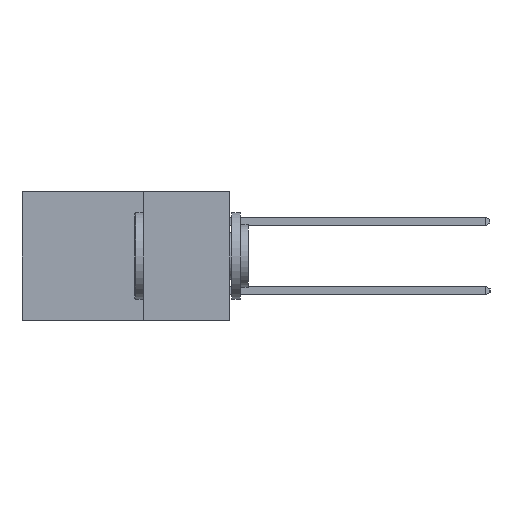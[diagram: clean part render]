
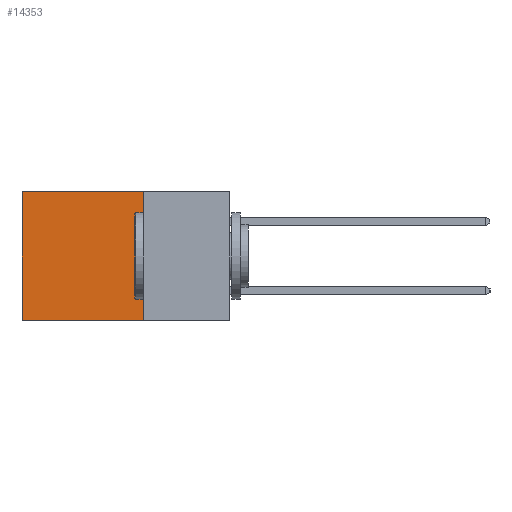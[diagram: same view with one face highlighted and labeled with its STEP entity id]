
A CAD part, left-side view. The second image highlights one B-rep face of the part: STEP entity #14353.
In plain terms, the highlighted planar face has unit normal (-1, 0, 0).
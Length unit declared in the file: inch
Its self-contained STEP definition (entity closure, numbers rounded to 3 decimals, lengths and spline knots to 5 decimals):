
#50 = ORIENTED_EDGE ( 'NONE', *, *, #10143, .T. ) ;
#382 = VECTOR ( 'NONE', #13634, 39.37008 ) ;
#398 = VECTOR ( 'NONE', #5019, 39.37008 ) ;
#512 = CARTESIAN_POINT ( 'NONE',  ( 0.2615, 0.6, -0.37 ) ) ;
#1094 = VECTOR ( 'NONE', #5701, 39.37008 ) ;
#2653 = ORIENTED_EDGE ( 'NONE', *, *, #5101, .F. ) ;
#3463 = CARTESIAN_POINT ( 'NONE',  ( 0.2615, 0.25, -0.37 ) ) ;
#4507 = FACE_OUTER_BOUND ( 'NONE', #9122, .T. ) ;
#4672 = VERTEX_POINT ( 'NONE', #5315 ) ;
#4679 = LINE ( 'NONE', #512, #382 ) ;
#5019 = DIRECTION ( 'NONE',  ( 0., 1., 0. ) ) ;
#5101 = EDGE_CURVE ( 'NONE', #6766, #11843, #14193, .T. ) ;
#5206 = DIRECTION ( 'NONE',  ( 0., 0., -1. ) ) ;
#5315 = CARTESIAN_POINT ( 'NONE',  ( 0.2615, 0.6, 0. ) ) ;
#5701 = DIRECTION ( 'NONE',  ( 0., 1., 0. ) ) ;
#6001 = CARTESIAN_POINT ( 'NONE',  ( 0.2615, 0.25, -0.37 ) ) ;
#6766 = VERTEX_POINT ( 'NONE', #3463 ) ;
#9122 = EDGE_LOOP ( 'NONE', ( #50, #2653, #11853, #18243 ) ) ;
#9210 = CARTESIAN_POINT ( 'NONE',  ( 0.2615, 0.25, -0.37 ) ) ;
#9922 = CARTESIAN_POINT ( 'NONE',  ( 0.2615, 0.25, 0. ) ) ;
#10143 = EDGE_CURVE ( 'NONE', #4672, #11843, #4679, .T. ) ;
#10268 = VECTOR ( 'NONE', #5206, 39.37008 ) ;
#10778 = LINE ( 'NONE', #15071, #10268 ) ;
#10846 = DIRECTION ( 'NONE',  ( 0., 0., -1. ) ) ;
#11432 = EDGE_CURVE ( 'NONE', #14646, #6766, #10778, .T. ) ;
#11843 = VERTEX_POINT ( 'NONE', #19402 ) ;
#11853 = ORIENTED_EDGE ( 'NONE', *, *, #11432, .F. ) ;
#13634 = DIRECTION ( 'NONE',  ( 0., 0., -1. ) ) ;
#14193 = LINE ( 'NONE', #6001, #1094 ) ;
#14353 = ADVANCED_FACE ( 'NONE', ( #4507 ), #20471, .F. ) ;
#14646 = VERTEX_POINT ( 'NONE', #9922 ) ;
#14897 = CARTESIAN_POINT ( 'NONE',  ( 0.2615, 0.25, 0. ) ) ;
#15071 = CARTESIAN_POINT ( 'NONE',  ( 0.2615, 0.25, -0.37 ) ) ;
#17262 = LINE ( 'NONE', #14897, #398 ) ;
#18243 = ORIENTED_EDGE ( 'NONE', *, *, #18936, .T. ) ;
#18936 = EDGE_CURVE ( 'NONE', #14646, #4672, #17262, .T. ) ;
#19402 = CARTESIAN_POINT ( 'NONE',  ( 0.2615, 0.6, -0.37 ) ) ;
#19752 = AXIS2_PLACEMENT_3D ( 'NONE', #9210, #20540, #10846 ) ;
#20471 = PLANE ( 'NONE',  #19752 ) ;
#20540 = DIRECTION ( 'NONE',  ( 1., 0., 0. ) ) ;
